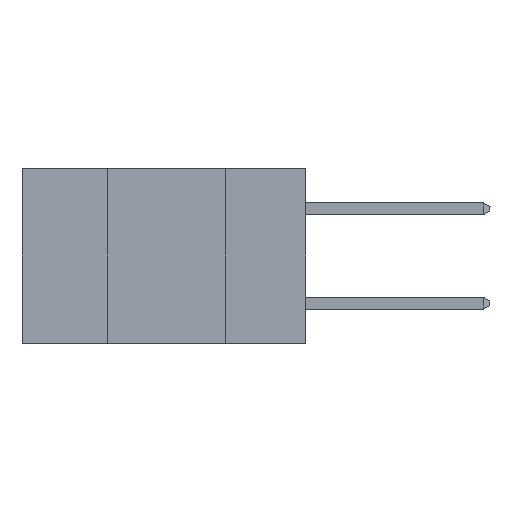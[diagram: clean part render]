
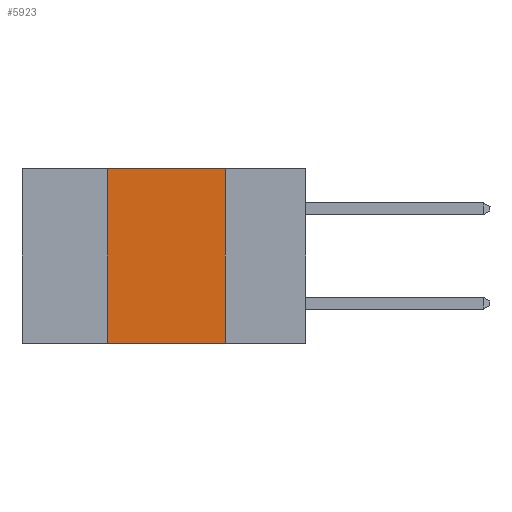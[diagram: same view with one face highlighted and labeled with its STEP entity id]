
A CAD part, left-side view. The second image highlights one B-rep face of the part: STEP entity #5923.
In plain terms, the highlighted planar face has unit normal (-1, 0, 0).
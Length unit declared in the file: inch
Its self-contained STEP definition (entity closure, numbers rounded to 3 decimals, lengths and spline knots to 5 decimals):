
#4161 = DIRECTION ( 'NONE',  ( 0., 0., -1. ) ) ;
#4519 = FACE_OUTER_BOUND ( 'NONE', #13925, .T. ) ;
#5062 = ORIENTED_EDGE ( 'NONE', *, *, #20618, .F. ) ;
#5185 = LINE ( 'NONE', #29997, #11045 ) ;
#5923 = ADVANCED_FACE ( 'NONE', ( #4519 ), #30316, .F. ) ;
#8117 = EDGE_CURVE ( 'NONE', #14734, #21438, #5185, .T. ) ;
#9083 = LINE ( 'NONE', #26912, #18135 ) ;
#9458 = VECTOR ( 'NONE', #14189, 39.37008 ) ;
#10476 = CARTESIAN_POINT ( 'NONE',  ( 0., 0.17, -0.37 ) ) ;
#10635 = CARTESIAN_POINT ( 'NONE',  ( 0., 0.42, -0.37 ) ) ;
#11045 = VECTOR ( 'NONE', #27606, 39.37008 ) ;
#12455 = VECTOR ( 'NONE', #30950, 39.37008 ) ;
#12494 = CARTESIAN_POINT ( 'NONE',  ( 0., 0.6, 0. ) ) ;
#13809 = CARTESIAN_POINT ( 'NONE',  ( 0., 0.42, 0. ) ) ;
#13925 = EDGE_LOOP ( 'NONE', ( #27212, #30870, #5062, #32424 ) ) ;
#14189 = DIRECTION ( 'NONE',  ( 0., 0., 1. ) ) ;
#14734 = VERTEX_POINT ( 'NONE', #10635 ) ;
#14797 = VERTEX_POINT ( 'NONE', #18552 ) ;
#14872 = EDGE_CURVE ( 'NONE', #14797, #21438, #9083, .T. ) ;
#15673 = CARTESIAN_POINT ( 'NONE',  ( 0., 0.6, 0. ) ) ;
#17580 = DIRECTION ( 'NONE',  ( 0., 0., -1. ) ) ;
#18135 = VECTOR ( 'NONE', #4161, 39.37008 ) ;
#18552 = CARTESIAN_POINT ( 'NONE',  ( 0., 0.17, 0. ) ) ;
#20136 = DIRECTION ( 'NONE',  ( 1., 0., 0. ) ) ;
#20618 = EDGE_CURVE ( 'NONE', #14734, #23561, #30792, .T. ) ;
#21365 = AXIS2_PLACEMENT_3D ( 'NONE', #12494, #20136, #17580 ) ;
#21438 = VERTEX_POINT ( 'NONE', #10476 ) ;
#22826 = EDGE_CURVE ( 'NONE', #23561, #14797, #24378, .T. ) ;
#23561 = VERTEX_POINT ( 'NONE', #13809 ) ;
#24378 = LINE ( 'NONE', #15673, #12455 ) ;
#26320 = CARTESIAN_POINT ( 'NONE',  ( 0., 0.42, 0. ) ) ;
#26912 = CARTESIAN_POINT ( 'NONE',  ( 0., 0.17, 0. ) ) ;
#27212 = ORIENTED_EDGE ( 'NONE', *, *, #14872, .F. ) ;
#27606 = DIRECTION ( 'NONE',  ( 0., -1., 0. ) ) ;
#29997 = CARTESIAN_POINT ( 'NONE',  ( 0., 0.6, -0.37 ) ) ;
#30316 = PLANE ( 'NONE',  #21365 ) ;
#30792 = LINE ( 'NONE', #26320, #9458 ) ;
#30870 = ORIENTED_EDGE ( 'NONE', *, *, #22826, .F. ) ;
#30950 = DIRECTION ( 'NONE',  ( 0., -1., 0. ) ) ;
#32424 = ORIENTED_EDGE ( 'NONE', *, *, #8117, .T. ) ;
